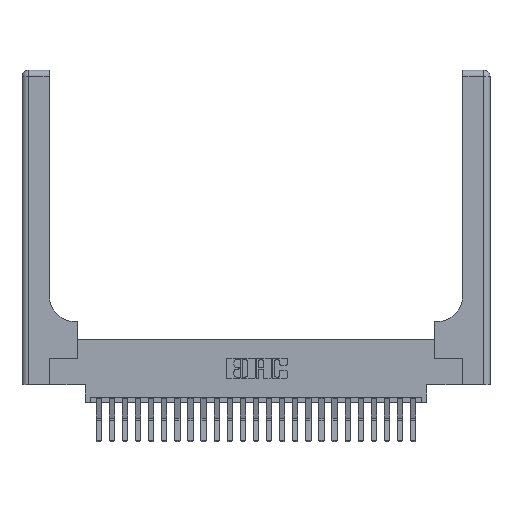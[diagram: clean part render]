
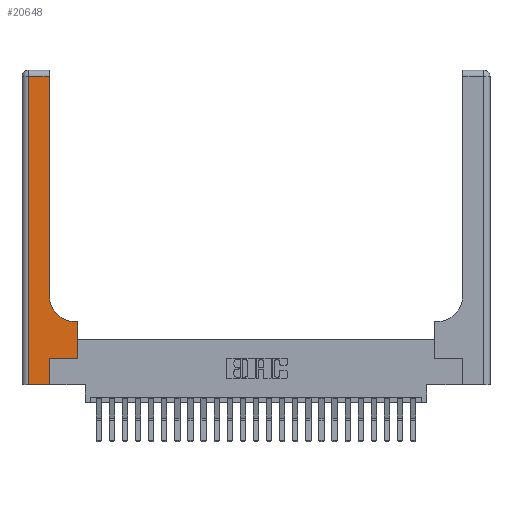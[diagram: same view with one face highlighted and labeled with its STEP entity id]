
A CAD part, top view. The second image highlights one B-rep face of the part: STEP entity #20648.
In plain terms, the highlighted planar face has unit normal (0, 0, 1).
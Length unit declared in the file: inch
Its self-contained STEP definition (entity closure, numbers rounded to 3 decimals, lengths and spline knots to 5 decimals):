
#138 = EDGE_CURVE ( 'NONE', #5006, #20611, #4891, .T. ) ;
#720 = VECTOR ( 'NONE', #20305, 39.37008 ) ;
#854 = CARTESIAN_POINT ( 'NONE',  ( 0.06, 0., 0.37 ) ) ;
#1068 = CARTESIAN_POINT ( 'NONE',  ( 0.26, 0.6, 0.37 ) ) ;
#1269 = EDGE_LOOP ( 'NONE', ( #3750, #13613, #4274, #20846, #19636, #8000, #12770, #9639, #10271 ) ) ;
#1458 = VECTOR ( 'NONE', #13148, 39.37008 ) ;
#1797 = DIRECTION ( 'NONE',  ( 0., -1., 0. ) ) ;
#1799 = DIRECTION ( 'NONE',  ( 1., 0., 0. ) ) ;
#1917 = CARTESIAN_POINT ( 'NONE',  ( 0.06, 3., 0.37 ) ) ;
#2461 = CARTESIAN_POINT ( 'NONE',  ( 0.265, 0., 0.37 ) ) ;
#2714 = DIRECTION ( 'NONE',  ( -1., 0., 0. ) ) ;
#2990 = EDGE_CURVE ( 'NONE', #11576, #16422, #24263, .T. ) ;
#3039 = CARTESIAN_POINT ( 'NONE',  ( 0., 0., 0.37 ) ) ;
#3562 = VECTOR ( 'NONE', #21163, 39.37008 ) ;
#3750 = ORIENTED_EDGE ( 'NONE', *, *, #17387, .T. ) ;
#4274 = ORIENTED_EDGE ( 'NONE', *, *, #6872, .T. ) ;
#4891 = LINE ( 'NONE', #3039, #9154 ) ;
#5006 = VERTEX_POINT ( 'NONE', #854 ) ;
#5241 = CARTESIAN_POINT ( 'NONE',  ( 0., 3., 0.37 ) ) ;
#5249 = LINE ( 'NONE', #11346, #17209 ) ;
#5363 = DIRECTION ( 'NONE',  ( -1., 0., 0. ) ) ;
#6537 = EDGE_CURVE ( 'NONE', #20611, #15312, #17457, .T. ) ;
#6561 = LINE ( 'NONE', #19687, #9689 ) ;
#6872 = EDGE_CURVE ( 'NONE', #17273, #5006, #21532, .T. ) ;
#7608 = LINE ( 'NONE', #13304, #18878 ) ;
#8000 = ORIENTED_EDGE ( 'NONE', *, *, #8723, .T. ) ;
#8723 = EDGE_CURVE ( 'NONE', #15312, #19325, #5249, .T. ) ;
#8863 = AXIS2_PLACEMENT_3D ( 'NONE', #19123, #12621, #22844 ) ;
#8964 = CARTESIAN_POINT ( 'NONE',  ( 0.51, 0.6, 0.37 ) ) ;
#9117 = VECTOR ( 'NONE', #1797, 39.37008 ) ;
#9154 = VECTOR ( 'NONE', #10626, 39.37008 ) ;
#9371 = EDGE_CURVE ( 'NONE', #21188, #17273, #6561, .T. ) ;
#9534 = CARTESIAN_POINT ( 'NONE',  ( 0.528, 0.25, 0.37 ) ) ;
#9639 = ORIENTED_EDGE ( 'NONE', *, *, #18736, .T. ) ;
#9689 = VECTOR ( 'NONE', #2714, 39.37008 ) ;
#10271 = ORIENTED_EDGE ( 'NONE', *, *, #2990, .T. ) ;
#10626 = DIRECTION ( 'NONE',  ( 1., 0., 0. ) ) ;
#10972 = PLANE ( 'NONE',  #12994 ) ;
#11014 = CARTESIAN_POINT ( 'NONE',  ( 0.265, 0.25, 0.37 ) ) ;
#11346 = CARTESIAN_POINT ( 'NONE',  ( 0.265, 0.25, 0.37 ) ) ;
#11576 = VERTEX_POINT ( 'NONE', #8964 ) ;
#12380 = CARTESIAN_POINT ( 'NONE',  ( 0.528, 0.6, 0.37 ) ) ;
#12621 = DIRECTION ( 'NONE',  ( 0., 0., -1. ) ) ;
#12770 = ORIENTED_EDGE ( 'NONE', *, *, #17995, .T. ) ;
#12889 = CARTESIAN_POINT ( 'NONE',  ( 0.26, 0.85, 0.37 ) ) ;
#12994 = AXIS2_PLACEMENT_3D ( 'NONE', #5241, #14797, #5363 ) ;
#12998 = LINE ( 'NONE', #20541, #720 ) ;
#13024 = LINE ( 'NONE', #1068, #1458 ) ;
#13148 = DIRECTION ( 'NONE',  ( -1., 0., 0. ) ) ;
#13304 = CARTESIAN_POINT ( 'NONE',  ( 0.26, 3., 0.37 ) ) ;
#13613 = ORIENTED_EDGE ( 'NONE', *, *, #9371, .T. ) ;
#14797 = DIRECTION ( 'NONE',  ( 0., 0., -1. ) ) ;
#15286 = DIRECTION ( 'NONE',  ( 0., 1., 0. ) ) ;
#15312 = VERTEX_POINT ( 'NONE', #11014 ) ;
#16422 = VERTEX_POINT ( 'NONE', #12889 ) ;
#17209 = VECTOR ( 'NONE', #1799, 39.37008 ) ;
#17273 = VERTEX_POINT ( 'NONE', #20480 ) ;
#17387 = EDGE_CURVE ( 'NONE', #16422, #21188, #7608, .T. ) ;
#17457 = LINE ( 'NONE', #2461, #3562 ) ;
#17995 = EDGE_CURVE ( 'NONE', #19325, #21421, #12998, .T. ) ;
#18736 = EDGE_CURVE ( 'NONE', #21421, #11576, #13024, .T. ) ;
#18878 = VECTOR ( 'NONE', #15286, 39.37008 ) ;
#19123 = CARTESIAN_POINT ( 'NONE',  ( 0.51, 0.85, 0.37 ) ) ;
#19325 = VERTEX_POINT ( 'NONE', #9534 ) ;
#19636 = ORIENTED_EDGE ( 'NONE', *, *, #6537, .T. ) ;
#19687 = CARTESIAN_POINT ( 'NONE',  ( 0., 2.94, 0.37 ) ) ;
#20305 = DIRECTION ( 'NONE',  ( 0., 1., 0. ) ) ;
#20480 = CARTESIAN_POINT ( 'NONE',  ( 0.06, 2.94, 0.37 ) ) ;
#20541 = CARTESIAN_POINT ( 'NONE',  ( 0.528, 0.25, 0.37 ) ) ;
#20611 = VERTEX_POINT ( 'NONE', #21497 ) ;
#20648 = ADVANCED_FACE ( 'NONE', ( #22215 ), #10972, .F. ) ;
#20846 = ORIENTED_EDGE ( 'NONE', *, *, #138, .T. ) ;
#21163 = DIRECTION ( 'NONE',  ( 0., 1., 0. ) ) ;
#21188 = VERTEX_POINT ( 'NONE', #23820 ) ;
#21421 = VERTEX_POINT ( 'NONE', #12380 ) ;
#21497 = CARTESIAN_POINT ( 'NONE',  ( 0.265, 0., 0.37 ) ) ;
#21532 = LINE ( 'NONE', #1917, #9117 ) ;
#22215 = FACE_OUTER_BOUND ( 'NONE', #1269, .T. ) ;
#22844 = DIRECTION ( 'NONE',  ( 1., 0., 0. ) ) ;
#23820 = CARTESIAN_POINT ( 'NONE',  ( 0.26, 2.94, 0.37 ) ) ;
#24263 = CIRCLE ( 'NONE', #8863, 0.25 ) ;
